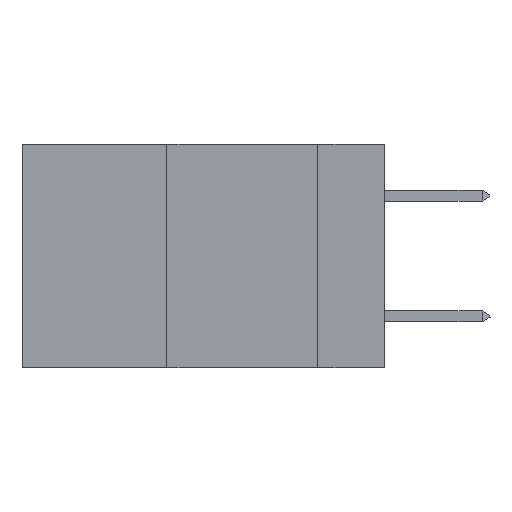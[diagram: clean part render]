
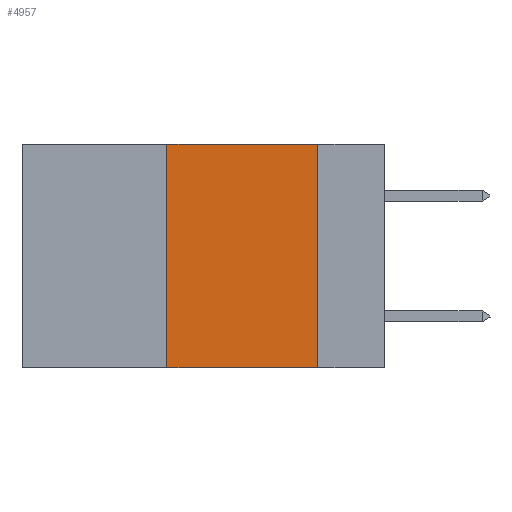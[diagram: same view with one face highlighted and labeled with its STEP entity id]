
A CAD part, left-side view. The second image highlights one B-rep face of the part: STEP entity #4957.
In plain terms, the highlighted planar face has unit normal (-1, 0, 0).
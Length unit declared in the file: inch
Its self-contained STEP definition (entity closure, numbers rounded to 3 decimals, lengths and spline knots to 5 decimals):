
#63 = EDGE_CURVE ( 'NONE', #13390, #6376, #6369, .T. ) ;
#98 = EDGE_CURVE ( 'NONE', #10087, #4656, #1706, .T. ) ;
#286 = DIRECTION ( 'NONE',  ( 0., -1., 0. ) ) ;
#499 = ORIENTED_EDGE ( 'NONE', *, *, #14398, .F. ) ;
#524 = CARTESIAN_POINT ( 'NONE',  ( 0., 0.6, 0. ) ) ;
#1706 = LINE ( 'NONE', #10843, #12684 ) ;
#1796 = ORIENTED_EDGE ( 'NONE', *, *, #6286, .F. ) ;
#2510 = PLANE ( 'NONE',  #8149 ) ;
#2702 = DIRECTION ( 'NONE',  ( 0., 0., -1. ) ) ;
#2753 = DIRECTION ( 'NONE',  ( 1., 0., 0. ) ) ;
#2961 = CARTESIAN_POINT ( 'NONE',  ( 0., 0.6, 0. ) ) ;
#3204 = CARTESIAN_POINT ( 'NONE',  ( 0., 0.36, 0. ) ) ;
#4656 = VERTEX_POINT ( 'NONE', #12657 ) ;
#4957 = ADVANCED_FACE ( 'NONE', ( #7309 ), #2510, .F. ) ;
#5179 = VECTOR ( 'NONE', #11887, 39.37008 ) ;
#5622 = LINE ( 'NONE', #3204, #5179 ) ;
#6199 = ORIENTED_EDGE ( 'NONE', *, *, #98, .T. ) ;
#6286 = EDGE_CURVE ( 'NONE', #6376, #4656, #7966, .T. ) ;
#6369 = LINE ( 'NONE', #524, #16775 ) ;
#6376 = VERTEX_POINT ( 'NONE', #7571 ) ;
#7309 = FACE_OUTER_BOUND ( 'NONE', #8179, .T. ) ;
#7571 = CARTESIAN_POINT ( 'NONE',  ( 0., 0.11, 0. ) ) ;
#7682 = ORIENTED_EDGE ( 'NONE', *, *, #63, .F. ) ;
#7966 = LINE ( 'NONE', #10291, #15177 ) ;
#8149 = AXIS2_PLACEMENT_3D ( 'NONE', #2961, #2753, #2702 ) ;
#8179 = EDGE_LOOP ( 'NONE', ( #1796, #7682, #499, #6199 ) ) ;
#10087 = VERTEX_POINT ( 'NONE', #14127 ) ;
#10291 = CARTESIAN_POINT ( 'NONE',  ( 0., 0.11, 0. ) ) ;
#10843 = CARTESIAN_POINT ( 'NONE',  ( 0., 0.6, -0.37 ) ) ;
#11887 = DIRECTION ( 'NONE',  ( 0., 0., 1. ) ) ;
#12040 = CARTESIAN_POINT ( 'NONE',  ( 0., 0.36, 0. ) ) ;
#12657 = CARTESIAN_POINT ( 'NONE',  ( 0., 0.11, -0.37 ) ) ;
#12684 = VECTOR ( 'NONE', #18044, 39.37008 ) ;
#13390 = VERTEX_POINT ( 'NONE', #12040 ) ;
#14127 = CARTESIAN_POINT ( 'NONE',  ( 0., 0.36, -0.37 ) ) ;
#14398 = EDGE_CURVE ( 'NONE', #10087, #13390, #5622, .T. ) ;
#15177 = VECTOR ( 'NONE', #15880, 39.37008 ) ;
#15880 = DIRECTION ( 'NONE',  ( 0., 0., -1. ) ) ;
#16775 = VECTOR ( 'NONE', #286, 39.37008 ) ;
#18044 = DIRECTION ( 'NONE',  ( 0., -1., 0. ) ) ;
